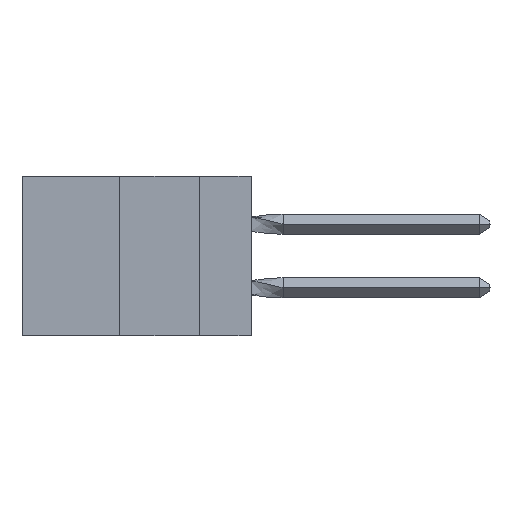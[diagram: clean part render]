
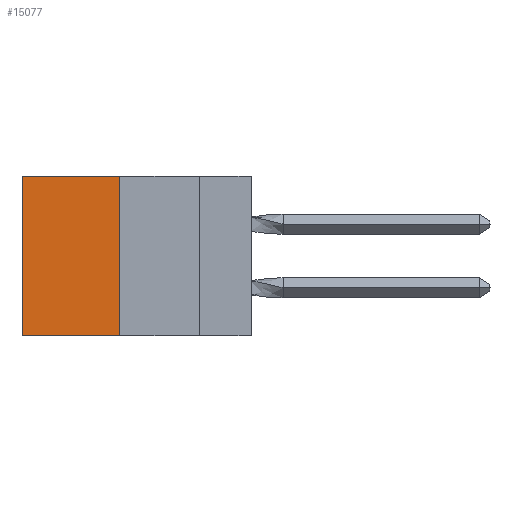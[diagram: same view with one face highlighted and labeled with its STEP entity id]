
A CAD part, left-side view. The second image highlights one B-rep face of the part: STEP entity #15077.
In plain terms, the highlighted planar face has unit normal (-1, 0, 0).
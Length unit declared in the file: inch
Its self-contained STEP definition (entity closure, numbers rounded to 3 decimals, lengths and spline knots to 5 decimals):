
#1443 = VECTOR ( 'NONE', #27145, 39.37008 ) ;
#1730 = VERTEX_POINT ( 'NONE', #21689 ) ;
#2047 = DIRECTION ( 'NONE',  ( 0., 0., -1. ) ) ;
#2310 = VERTEX_POINT ( 'NONE', #23141 ) ;
#4400 = PLANE ( 'NONE',  #21117 ) ;
#4621 = EDGE_CURVE ( 'NONE', #1730, #27574, #29393, .T. ) ;
#5528 = LINE ( 'NONE', #32970, #16453 ) ;
#8401 = LINE ( 'NONE', #24415, #15660 ) ;
#9722 = DIRECTION ( 'NONE',  ( 1., 0., 0. ) ) ;
#10822 = CARTESIAN_POINT ( 'NONE',  ( 0.305, 0.413, 0. ) ) ;
#11368 = CARTESIAN_POINT ( 'NONE',  ( 0.305, 0.413, -0.5 ) ) ;
#11386 = CARTESIAN_POINT ( 'NONE',  ( 0.305, 0.413, -0.5 ) ) ;
#14109 = ORIENTED_EDGE ( 'NONE', *, *, #30368, .T. ) ;
#14422 = EDGE_CURVE ( 'NONE', #27574, #2310, #8401, .T. ) ;
#15077 = ADVANCED_FACE ( 'NONE', ( #27375 ), #4400, .F. ) ;
#15660 = VECTOR ( 'NONE', #16965, 39.37008 ) ;
#15945 = LINE ( 'NONE', #10822, #32589 ) ;
#16453 = VECTOR ( 'NONE', #22732, 39.37008 ) ;
#16965 = DIRECTION ( 'NONE',  ( 0., 1., 0. ) ) ;
#18486 = ORIENTED_EDGE ( 'NONE', *, *, #32795, .T. ) ;
#20011 = CARTESIAN_POINT ( 'NONE',  ( 0.305, 0.413, -0.5 ) ) ;
#21117 = AXIS2_PLACEMENT_3D ( 'NONE', #20011, #9722, #2047 ) ;
#21211 = DIRECTION ( 'NONE',  ( 0., 1., 0. ) ) ;
#21340 = CARTESIAN_POINT ( 'NONE',  ( 0.305, 0.72, 0. ) ) ;
#21689 = CARTESIAN_POINT ( 'NONE',  ( 0.305, 0.413, 0. ) ) ;
#22029 = ORIENTED_EDGE ( 'NONE', *, *, #14422, .F. ) ;
#22732 = DIRECTION ( 'NONE',  ( 0., 0., -1. ) ) ;
#23141 = CARTESIAN_POINT ( 'NONE',  ( 0.305, 0.72, -0.5 ) ) ;
#24415 = CARTESIAN_POINT ( 'NONE',  ( 0.305, 0.413, -0.5 ) ) ;
#27145 = DIRECTION ( 'NONE',  ( 0., 0., -1. ) ) ;
#27375 = FACE_OUTER_BOUND ( 'NONE', #29668, .T. ) ;
#27574 = VERTEX_POINT ( 'NONE', #11368 ) ;
#29393 = LINE ( 'NONE', #11386, #1443 ) ;
#29668 = EDGE_LOOP ( 'NONE', ( #14109, #22029, #32568, #18486 ) ) ;
#30368 = EDGE_CURVE ( 'NONE', #31194, #2310, #5528, .T. ) ;
#31194 = VERTEX_POINT ( 'NONE', #21340 ) ;
#32568 = ORIENTED_EDGE ( 'NONE', *, *, #4621, .F. ) ;
#32589 = VECTOR ( 'NONE', #21211, 39.37008 ) ;
#32795 = EDGE_CURVE ( 'NONE', #1730, #31194, #15945, .T. ) ;
#32970 = CARTESIAN_POINT ( 'NONE',  ( 0.305, 0.72, -0.5 ) ) ;
